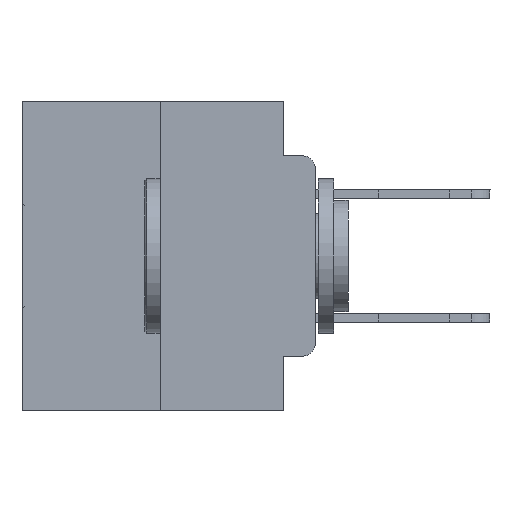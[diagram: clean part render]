
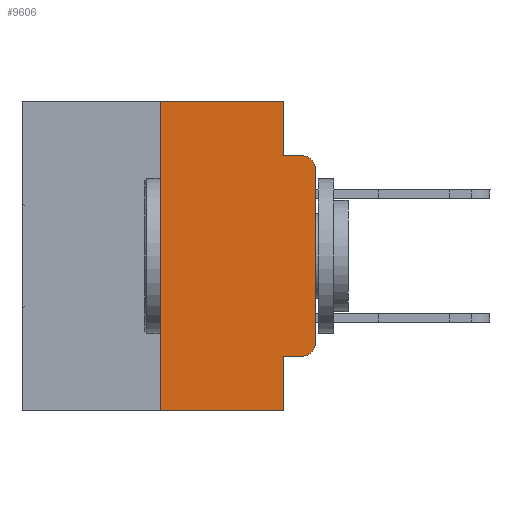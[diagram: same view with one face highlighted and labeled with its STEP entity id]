
A CAD part, left-side view. The second image highlights one B-rep face of the part: STEP entity #9606.
In plain terms, the highlighted planar face has unit normal (-1, 0, 0).
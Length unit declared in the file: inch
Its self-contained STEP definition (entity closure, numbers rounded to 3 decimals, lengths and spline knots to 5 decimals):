
#75 = DIRECTION ( 'NONE',  ( 0., -1., 0. ) ) ;
#182 = CARTESIAN_POINT ( 'NONE',  ( 0., 0., -0.3915 ) ) ;
#463 = VECTOR ( 'NONE', #2318, 39.37008 ) ;
#538 = LINE ( 'NONE', #29625, #23495 ) ;
#886 = VECTOR ( 'NONE', #30610, 39.37008 ) ;
#1128 = DIRECTION ( 'NONE',  ( 0., 0., 1. ) ) ;
#1723 = EDGE_CURVE ( 'NONE', #21530, #15586, #8612, .T. ) ;
#2318 = DIRECTION ( 'NONE',  ( 0., -1., 0. ) ) ;
#2630 = LINE ( 'NONE', #7155, #463 ) ;
#2736 = CARTESIAN_POINT ( 'NONE',  ( 0., 0.25, -0.5 ) ) ;
#4464 = VECTOR ( 'NONE', #1128, 39.37008 ) ;
#4557 = LINE ( 'NONE', #18371, #22324 ) ;
#4683 = CARTESIAN_POINT ( 'NONE',  ( 0., 0.02, -0.0885 ) ) ;
#4779 = CARTESIAN_POINT ( 'NONE',  ( 0., 0.051, -0.5 ) ) ;
#5006 = EDGE_CURVE ( 'NONE', #24184, #12546, #24019, .T. ) ;
#5533 = VERTEX_POINT ( 'NONE', #29595 ) ;
#5705 = AXIS2_PLACEMENT_3D ( 'NONE', #18917, #21096, #15982 ) ;
#6133 = LINE ( 'NONE', #8303, #4464 ) ;
#6166 = ORIENTED_EDGE ( 'NONE', *, *, #12125, .T. ) ;
#6842 = CARTESIAN_POINT ( 'NONE',  ( 0., 0.02, -0.4115 ) ) ;
#6872 = ORIENTED_EDGE ( 'NONE', *, *, #9608, .T. ) ;
#6907 = VECTOR ( 'NONE', #75, 39.37008 ) ;
#7155 = CARTESIAN_POINT ( 'NONE',  ( 0., 0.051, -0.0885 ) ) ;
#7348 = ORIENTED_EDGE ( 'NONE', *, *, #25205, .T. ) ;
#7575 = VERTEX_POINT ( 'NONE', #15814 ) ;
#8303 = CARTESIAN_POINT ( 'NONE',  ( 0., 0.25, 0. ) ) ;
#8612 = CIRCLE ( 'NONE', #24471, 0.02 ) ;
#9424 = CARTESIAN_POINT ( 'NONE',  ( 0., 0.473, 0. ) ) ;
#9526 = EDGE_CURVE ( 'NONE', #22101, #16148, #6133, .T. ) ;
#9606 = ADVANCED_FACE ( 'NONE', ( #13713 ), #13873, .F. ) ;
#9608 = EDGE_CURVE ( 'NONE', #22101, #12546, #4557, .T. ) ;
#10237 = LINE ( 'NONE', #19677, #16584 ) ;
#10278 = VERTEX_POINT ( 'NONE', #4683 ) ;
#10284 = EDGE_LOOP ( 'NONE', ( #7348, #14100, #15273, #23834, #19335, #29491, #6872, #30020, #6166, #28368 ) ) ;
#10631 = DIRECTION ( 'NONE',  ( 0., 0., -1. ) ) ;
#11083 = CARTESIAN_POINT ( 'NONE',  ( 0., 0.02, -0.3915 ) ) ;
#11395 = DIRECTION ( 'NONE',  ( 0., -1., 0. ) ) ;
#12125 = EDGE_CURVE ( 'NONE', #24184, #21530, #10237, .T. ) ;
#12546 = VERTEX_POINT ( 'NONE', #4779 ) ;
#13713 = FACE_OUTER_BOUND ( 'NONE', #10284, .T. ) ;
#13794 = LINE ( 'NONE', #15974, #886 ) ;
#13873 = PLANE ( 'NONE',  #14891 ) ;
#14100 = ORIENTED_EDGE ( 'NONE', *, *, #26353, .T. ) ;
#14891 = AXIS2_PLACEMENT_3D ( 'NONE', #30223, #27725, #16197 ) ;
#15151 = DIRECTION ( 'NONE',  ( -1., 0., 0. ) ) ;
#15273 = ORIENTED_EDGE ( 'NONE', *, *, #19069, .F. ) ;
#15586 = VERTEX_POINT ( 'NONE', #182 ) ;
#15814 = CARTESIAN_POINT ( 'NONE',  ( 0., 0.051, -0.0885 ) ) ;
#15974 = CARTESIAN_POINT ( 'NONE',  ( 0., 0.051, 0. ) ) ;
#15982 = DIRECTION ( 'NONE',  ( 0., 0., -1. ) ) ;
#16148 = VERTEX_POINT ( 'NONE', #27189 ) ;
#16197 = DIRECTION ( 'NONE',  ( 0., 0., -1. ) ) ;
#16389 = EDGE_CURVE ( 'NONE', #5533, #7575, #13794, .T. ) ;
#16584 = VECTOR ( 'NONE', #21887, 39.37008 ) ;
#16928 = EDGE_CURVE ( 'NONE', #16148, #5533, #30738, .T. ) ;
#16975 = CARTESIAN_POINT ( 'NONE',  ( 0., 0., -0.1085 ) ) ;
#18371 = CARTESIAN_POINT ( 'NONE',  ( 0., 0.473, -0.5 ) ) ;
#18917 = CARTESIAN_POINT ( 'NONE',  ( 0., 0.02, -0.1085 ) ) ;
#19069 = EDGE_CURVE ( 'NONE', #7575, #10278, #2630, .T. ) ;
#19335 = ORIENTED_EDGE ( 'NONE', *, *, #16928, .F. ) ;
#19677 = CARTESIAN_POINT ( 'NONE',  ( 0., 0.051, -0.4115 ) ) ;
#20087 = VECTOR ( 'NONE', #25471, 39.37008 ) ;
#21096 = DIRECTION ( 'NONE',  ( -1., 0., 0. ) ) ;
#21530 = VERTEX_POINT ( 'NONE', #6842 ) ;
#21887 = DIRECTION ( 'NONE',  ( 0., -1., 0. ) ) ;
#22101 = VERTEX_POINT ( 'NONE', #2736 ) ;
#22324 = VECTOR ( 'NONE', #11395, 39.37008 ) ;
#23293 = CARTESIAN_POINT ( 'NONE',  ( 0., 0.051, 0. ) ) ;
#23495 = VECTOR ( 'NONE', #29322, 39.37008 ) ;
#23834 = ORIENTED_EDGE ( 'NONE', *, *, #16389, .F. ) ;
#24019 = LINE ( 'NONE', #23293, #20087 ) ;
#24184 = VERTEX_POINT ( 'NONE', #27883 ) ;
#24471 = AXIS2_PLACEMENT_3D ( 'NONE', #11083, #15151, #10631 ) ;
#24540 = CIRCLE ( 'NONE', #5705, 0.02 ) ;
#25205 = EDGE_CURVE ( 'NONE', #15586, #26865, #538, .T. ) ;
#25471 = DIRECTION ( 'NONE',  ( 0., 0., -1. ) ) ;
#26353 = EDGE_CURVE ( 'NONE', #26865, #10278, #24540, .T. ) ;
#26865 = VERTEX_POINT ( 'NONE', #16975 ) ;
#27189 = CARTESIAN_POINT ( 'NONE',  ( 0., 0.25, 0. ) ) ;
#27725 = DIRECTION ( 'NONE',  ( 1., 0., 0. ) ) ;
#27883 = CARTESIAN_POINT ( 'NONE',  ( 0., 0.051, -0.4115 ) ) ;
#28368 = ORIENTED_EDGE ( 'NONE', *, *, #1723, .T. ) ;
#29322 = DIRECTION ( 'NONE',  ( 0., 0., 1. ) ) ;
#29491 = ORIENTED_EDGE ( 'NONE', *, *, #9526, .F. ) ;
#29595 = CARTESIAN_POINT ( 'NONE',  ( 0., 0.051, 0. ) ) ;
#29625 = CARTESIAN_POINT ( 'NONE',  ( 0., 0., 0. ) ) ;
#30020 = ORIENTED_EDGE ( 'NONE', *, *, #5006, .F. ) ;
#30223 = CARTESIAN_POINT ( 'NONE',  ( 0., 0.473, 0. ) ) ;
#30610 = DIRECTION ( 'NONE',  ( 0., 0., -1. ) ) ;
#30738 = LINE ( 'NONE', #9424, #6907 ) ;
